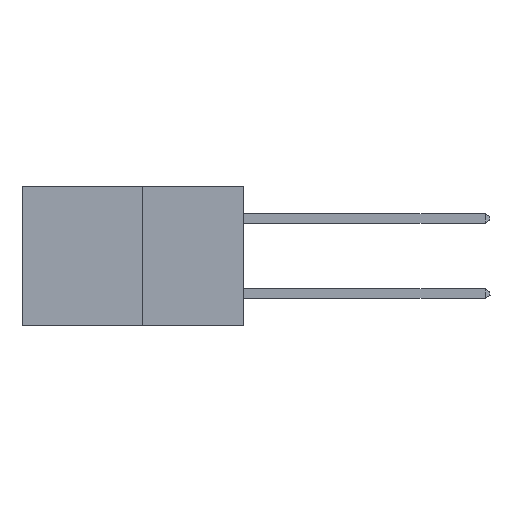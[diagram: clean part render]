
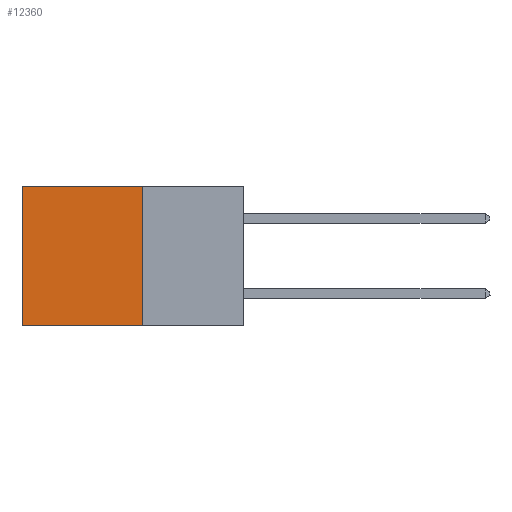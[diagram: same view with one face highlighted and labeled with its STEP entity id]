
A CAD part, left-side view. The second image highlights one B-rep face of the part: STEP entity #12360.
In plain terms, the highlighted planar face has unit normal (-1, 0, 0).
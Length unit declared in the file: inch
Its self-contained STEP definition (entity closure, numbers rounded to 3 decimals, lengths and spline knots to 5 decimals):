
#117 = DIRECTION ( 'NONE',  ( 0., 0., -1. ) ) ;
#753 = CARTESIAN_POINT ( 'NONE',  ( 0.277, 0.27, 0. ) ) ;
#905 = VERTEX_POINT ( 'NONE', #13230 ) ;
#1484 = LINE ( 'NONE', #12916, #4186 ) ;
#1763 = AXIS2_PLACEMENT_3D ( 'NONE', #4429, #13497, #6825 ) ;
#2025 = DIRECTION ( 'NONE',  ( 0., 1., 0. ) ) ;
#2198 = CARTESIAN_POINT ( 'NONE',  ( 0.277, 0.27, -0.37 ) ) ;
#2836 = ORIENTED_EDGE ( 'NONE', *, *, #7670, .F. ) ;
#3140 = EDGE_CURVE ( 'NONE', #12254, #8628, #1484, .T. ) ;
#3444 = ORIENTED_EDGE ( 'NONE', *, *, #7974, .T. ) ;
#3997 = VECTOR ( 'NONE', #11045, 39.37008 ) ;
#4186 = VECTOR ( 'NONE', #117, 39.37008 ) ;
#4429 = CARTESIAN_POINT ( 'NONE',  ( 0.277, 0.27, -0.37 ) ) ;
#4691 = LINE ( 'NONE', #7544, #10438 ) ;
#4998 = ORIENTED_EDGE ( 'NONE', *, *, #3140, .F. ) ;
#6355 = LINE ( 'NONE', #2198, #12004 ) ;
#6364 = EDGE_CURVE ( 'NONE', #905, #10208, #12726, .T. ) ;
#6825 = DIRECTION ( 'NONE',  ( 0., 0., -1. ) ) ;
#7544 = CARTESIAN_POINT ( 'NONE',  ( 0.277, 0.27, 0. ) ) ;
#7670 = EDGE_CURVE ( 'NONE', #8628, #10208, #6355, .T. ) ;
#7974 = EDGE_CURVE ( 'NONE', #12254, #905, #4691, .T. ) ;
#8628 = VERTEX_POINT ( 'NONE', #12021 ) ;
#10208 = VERTEX_POINT ( 'NONE', #13350 ) ;
#10438 = VECTOR ( 'NONE', #12036, 39.37008 ) ;
#11045 = DIRECTION ( 'NONE',  ( 0., 0., -1. ) ) ;
#11095 = CARTESIAN_POINT ( 'NONE',  ( 0.277, 0.59, -0.37 ) ) ;
#12004 = VECTOR ( 'NONE', #2025, 39.37008 ) ;
#12021 = CARTESIAN_POINT ( 'NONE',  ( 0.277, 0.27, -0.37 ) ) ;
#12036 = DIRECTION ( 'NONE',  ( 0., 1., 0. ) ) ;
#12254 = VERTEX_POINT ( 'NONE', #753 ) ;
#12277 = ORIENTED_EDGE ( 'NONE', *, *, #6364, .T. ) ;
#12360 = ADVANCED_FACE ( 'NONE', ( #14218 ), #12402, .F. ) ;
#12402 = PLANE ( 'NONE',  #1763 ) ;
#12512 = EDGE_LOOP ( 'NONE', ( #12277, #2836, #4998, #3444 ) ) ;
#12726 = LINE ( 'NONE', #11095, #3997 ) ;
#12916 = CARTESIAN_POINT ( 'NONE',  ( 0.277, 0.27, -0.37 ) ) ;
#13230 = CARTESIAN_POINT ( 'NONE',  ( 0.277, 0.59, 0. ) ) ;
#13350 = CARTESIAN_POINT ( 'NONE',  ( 0.277, 0.59, -0.37 ) ) ;
#13497 = DIRECTION ( 'NONE',  ( 1., 0., 0. ) ) ;
#14218 = FACE_OUTER_BOUND ( 'NONE', #12512, .T. ) ;
